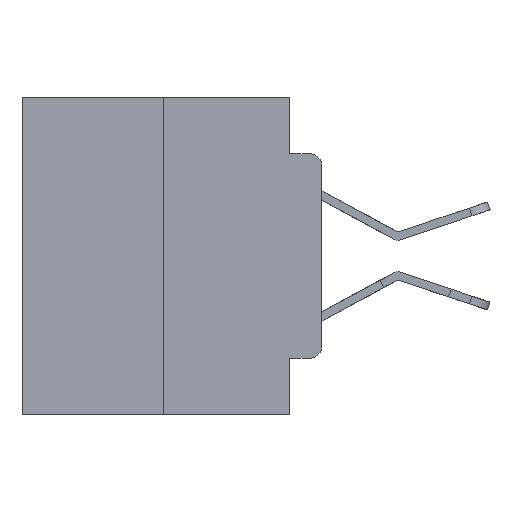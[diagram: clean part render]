
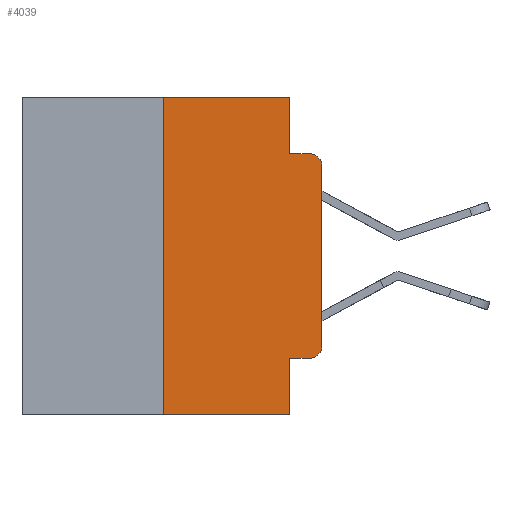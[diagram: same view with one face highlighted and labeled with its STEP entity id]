
A CAD part, left-side view. The second image highlights one B-rep face of the part: STEP entity #4039.
In plain terms, the highlighted planar face has unit normal (-1, 0, 0).
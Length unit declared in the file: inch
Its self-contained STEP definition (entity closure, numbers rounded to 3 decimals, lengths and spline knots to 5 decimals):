
#254 = VERTEX_POINT ( 'NONE', #435 ) ;
#288 = ORIENTED_EDGE ( 'NONE', *, *, #2861, .F. ) ;
#298 = CARTESIAN_POINT ( 'NONE',  ( 0., 0.051, -0.0885 ) ) ;
#377 = CARTESIAN_POINT ( 'NONE',  ( 0., 0.473, 0. ) ) ;
#435 = CARTESIAN_POINT ( 'NONE',  ( 0., 0.051, 0. ) ) ;
#673 = CARTESIAN_POINT ( 'NONE',  ( 0., 0.02, -0.4115 ) ) ;
#1035 = DIRECTION ( 'NONE',  ( 0., 0., -1. ) ) ;
#1210 = AXIS2_PLACEMENT_3D ( 'NONE', #19504, #2364, #2538 ) ;
#1328 = ORIENTED_EDGE ( 'NONE', *, *, #26571, .F. ) ;
#1422 = EDGE_CURVE ( 'NONE', #254, #20928, #18627, .T. ) ;
#1958 = LINE ( 'NONE', #11196, #23296 ) ;
#2164 = LINE ( 'NONE', #377, #13341 ) ;
#2364 = DIRECTION ( 'NONE',  ( -1., 0., 0. ) ) ;
#2517 = DIRECTION ( 'NONE',  ( 0., 0., -1. ) ) ;
#2538 = DIRECTION ( 'NONE',  ( 0., 0., -1. ) ) ;
#2610 = DIRECTION ( 'NONE',  ( -1., 0., 0. ) ) ;
#2694 = CARTESIAN_POINT ( 'NONE',  ( 0., 0.02, -0.3915 ) ) ;
#2811 = CIRCLE ( 'NONE', #24267, 0.02 ) ;
#2861 = EDGE_CURVE ( 'NONE', #20928, #10528, #1958, .T. ) ;
#2879 = ORIENTED_EDGE ( 'NONE', *, *, #10503, .F. ) ;
#2927 = CARTESIAN_POINT ( 'NONE',  ( 0., 0.051, -0.5 ) ) ;
#3205 = PLANE ( 'NONE',  #22375 ) ;
#3885 = VERTEX_POINT ( 'NONE', #2927 ) ;
#4039 = ADVANCED_FACE ( 'NONE', ( #7864 ), #3205, .F. ) ;
#4190 = DIRECTION ( 'NONE',  ( 0., 0., 1. ) ) ;
#4757 = CARTESIAN_POINT ( 'NONE',  ( 0., 0., -0.1085 ) ) ;
#4948 = VECTOR ( 'NONE', #9242, 39.37008 ) ;
#5353 = LINE ( 'NONE', #23455, #21176 ) ;
#5728 = EDGE_CURVE ( 'NONE', #6217, #10528, #16873, .T. ) ;
#6131 = DIRECTION ( 'NONE',  ( 0., 0., -1. ) ) ;
#6217 = VERTEX_POINT ( 'NONE', #4757 ) ;
#6272 = EDGE_CURVE ( 'NONE', #14123, #16222, #2811, .T. ) ;
#7622 = ORIENTED_EDGE ( 'NONE', *, *, #1422, .F. ) ;
#7864 = FACE_OUTER_BOUND ( 'NONE', #26013, .T. ) ;
#8350 = CARTESIAN_POINT ( 'NONE',  ( 0., 0., -0.3915 ) ) ;
#8361 = VECTOR ( 'NONE', #17819, 39.37008 ) ;
#8785 = CARTESIAN_POINT ( 'NONE',  ( 0., 0., 0. ) ) ;
#8858 = DIRECTION ( 'NONE',  ( 0., -1., 0. ) ) ;
#8861 = ORIENTED_EDGE ( 'NONE', *, *, #11851, .F. ) ;
#9084 = EDGE_CURVE ( 'NONE', #24989, #14123, #5353, .T. ) ;
#9242 = DIRECTION ( 'NONE',  ( 0., -1., 0. ) ) ;
#10503 = EDGE_CURVE ( 'NONE', #24989, #3885, #11513, .T. ) ;
#10528 = VERTEX_POINT ( 'NONE', #12432 ) ;
#10583 = LINE ( 'NONE', #23512, #4948 ) ;
#10637 = ORIENTED_EDGE ( 'NONE', *, *, #5728, .T. ) ;
#11196 = CARTESIAN_POINT ( 'NONE',  ( 0., 0.051, -0.0885 ) ) ;
#11513 = LINE ( 'NONE', #20532, #16334 ) ;
#11851 = EDGE_CURVE ( 'NONE', #18178, #13192, #25704, .T. ) ;
#12175 = ORIENTED_EDGE ( 'NONE', *, *, #9084, .T. ) ;
#12432 = CARTESIAN_POINT ( 'NONE',  ( 0., 0.02, -0.0885 ) ) ;
#12746 = EDGE_CURVE ( 'NONE', #16222, #6217, #15401, .T. ) ;
#13192 = VERTEX_POINT ( 'NONE', #26447 ) ;
#13341 = VECTOR ( 'NONE', #8858, 39.37008 ) ;
#14077 = CARTESIAN_POINT ( 'NONE',  ( 0., 0.051, -0.4115 ) ) ;
#14123 = VERTEX_POINT ( 'NONE', #673 ) ;
#15390 = ORIENTED_EDGE ( 'NONE', *, *, #12746, .T. ) ;
#15401 = LINE ( 'NONE', #8785, #21418 ) ;
#15627 = VECTOR ( 'NONE', #4190, 39.37008 ) ;
#15724 = DIRECTION ( 'NONE',  ( 1., 0., 0. ) ) ;
#16222 = VERTEX_POINT ( 'NONE', #8350 ) ;
#16334 = VECTOR ( 'NONE', #6131, 39.37008 ) ;
#16873 = CIRCLE ( 'NONE', #1210, 0.02 ) ;
#17819 = DIRECTION ( 'NONE',  ( 0., 0., -1. ) ) ;
#18098 = DIRECTION ( 'NONE',  ( 0., -1., 0. ) ) ;
#18178 = VERTEX_POINT ( 'NONE', #26150 ) ;
#18506 = CARTESIAN_POINT ( 'NONE',  ( 0., 0.051, 0. ) ) ;
#18627 = LINE ( 'NONE', #18506, #8361 ) ;
#18681 = CARTESIAN_POINT ( 'NONE',  ( 0., 0.25, 0. ) ) ;
#19504 = CARTESIAN_POINT ( 'NONE',  ( 0., 0.02, -0.1085 ) ) ;
#20532 = CARTESIAN_POINT ( 'NONE',  ( 0., 0.051, 0. ) ) ;
#20928 = VERTEX_POINT ( 'NONE', #298 ) ;
#21123 = ORIENTED_EDGE ( 'NONE', *, *, #6272, .T. ) ;
#21176 = VECTOR ( 'NONE', #25462, 39.37008 ) ;
#21418 = VECTOR ( 'NONE', #24986, 39.37008 ) ;
#21791 = EDGE_CURVE ( 'NONE', #18178, #3885, #10583, .T. ) ;
#21807 = CARTESIAN_POINT ( 'NONE',  ( 0., 0.473, 0. ) ) ;
#22375 = AXIS2_PLACEMENT_3D ( 'NONE', #21807, #15724, #1035 ) ;
#23296 = VECTOR ( 'NONE', #18098, 39.37008 ) ;
#23455 = CARTESIAN_POINT ( 'NONE',  ( 0., 0.051, -0.4115 ) ) ;
#23512 = CARTESIAN_POINT ( 'NONE',  ( 0., 0.473, -0.5 ) ) ;
#24267 = AXIS2_PLACEMENT_3D ( 'NONE', #2694, #2610, #2517 ) ;
#24986 = DIRECTION ( 'NONE',  ( 0., 0., 1. ) ) ;
#24989 = VERTEX_POINT ( 'NONE', #14077 ) ;
#25462 = DIRECTION ( 'NONE',  ( 0., -1., 0. ) ) ;
#25704 = LINE ( 'NONE', #18681, #15627 ) ;
#26013 = EDGE_LOOP ( 'NONE', ( #15390, #10637, #288, #7622, #1328, #8861, #26579, #2879, #12175, #21123 ) ) ;
#26150 = CARTESIAN_POINT ( 'NONE',  ( 0., 0.25, -0.5 ) ) ;
#26447 = CARTESIAN_POINT ( 'NONE',  ( 0., 0.25, 0. ) ) ;
#26571 = EDGE_CURVE ( 'NONE', #13192, #254, #2164, .T. ) ;
#26579 = ORIENTED_EDGE ( 'NONE', *, *, #21791, .T. ) ;
